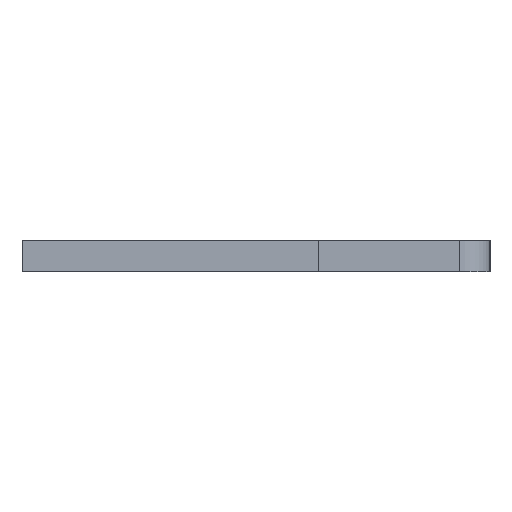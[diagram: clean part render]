
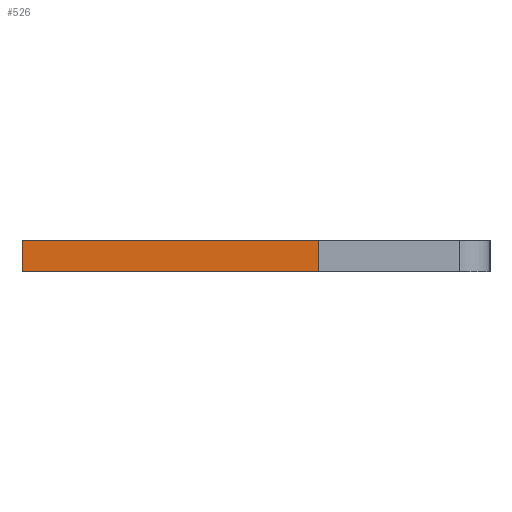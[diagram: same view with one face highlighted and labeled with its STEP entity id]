
A CAD part, left-side view. The second image highlights one B-rep face of the part: STEP entity #526.
In plain terms, the highlighted face is planar.
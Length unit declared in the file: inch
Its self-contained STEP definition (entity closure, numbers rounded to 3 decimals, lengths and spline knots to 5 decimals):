
#47 = ORIENTED_EDGE ( 'NONE', *, *, #707, .T. ) ;
#211 = CARTESIAN_POINT ( 'NONE',  ( 0.01, 0.15, -0.04 ) ) ;
#307 = LINE ( 'NONE', #580, #991 ) ;
#355 = DIRECTION ( 'NONE',  ( -1., 0., 0. ) ) ;
#461 = EDGE_CURVE ( 'NONE', #1667, #1750, #1270, .T. ) ;
#514 = LINE ( 'NONE', #666, #1450 ) ;
#526 = ADVANCED_FACE ( 'NONE', ( #1645 ), #1375, .F. ) ;
#580 = CARTESIAN_POINT ( 'NONE',  ( 0.01, -0.04, -0.04 ) ) ;
#611 = LINE ( 'NONE', #1779, #1661 ) ;
#666 = CARTESIAN_POINT ( 'NONE',  ( -0.01, 0.15, -0.04 ) ) ;
#679 = EDGE_LOOP ( 'NONE', ( #47, #1548, #1771, #1090 ) ) ;
#707 = EDGE_CURVE ( 'NONE', #1342, #1750, #514, .T. ) ;
#747 = DIRECTION ( 'NONE',  ( 0., 1., 0. ) ) ;
#776 = DIRECTION ( 'NONE',  ( 1., 0., 0. ) ) ;
#801 = DIRECTION ( 'NONE',  ( 0., 0., 1. ) ) ;
#887 = DIRECTION ( 'NONE',  ( -1., 0., 0. ) ) ;
#944 = VERTEX_POINT ( 'NONE', #1073 ) ;
#991 = VECTOR ( 'NONE', #887, 39.37008 ) ;
#1073 = CARTESIAN_POINT ( 'NONE',  ( 0.01, -0.04, -0.04 ) ) ;
#1090 = ORIENTED_EDGE ( 'NONE', *, *, #1600, .T. ) ;
#1099 = CARTESIAN_POINT ( 'NONE',  ( -0.01, -0.04, -0.04 ) ) ;
#1116 = EDGE_CURVE ( 'NONE', #944, #1667, #611, .T. ) ;
#1264 = DIRECTION ( 'NONE',  ( 0., 1., 0. ) ) ;
#1270 = LINE ( 'NONE', #211, #1506 ) ;
#1309 = AXIS2_PLACEMENT_3D ( 'NONE', #1521, #801, #776 ) ;
#1342 = VERTEX_POINT ( 'NONE', #1099 ) ;
#1375 = PLANE ( 'NONE',  #1309 ) ;
#1450 = VECTOR ( 'NONE', #1264, 39.37008 ) ;
#1470 = CARTESIAN_POINT ( 'NONE',  ( 0.01, 0.15, -0.04 ) ) ;
#1506 = VECTOR ( 'NONE', #355, 39.37008 ) ;
#1521 = CARTESIAN_POINT ( 'NONE',  ( 0.01, 0.15, -0.04 ) ) ;
#1548 = ORIENTED_EDGE ( 'NONE', *, *, #461, .F. ) ;
#1600 = EDGE_CURVE ( 'NONE', #944, #1342, #307, .T. ) ;
#1645 = FACE_OUTER_BOUND ( 'NONE', #679, .T. ) ;
#1661 = VECTOR ( 'NONE', #747, 39.37008 ) ;
#1667 = VERTEX_POINT ( 'NONE', #1470 ) ;
#1750 = VERTEX_POINT ( 'NONE', #1770 ) ;
#1770 = CARTESIAN_POINT ( 'NONE',  ( -0.01, 0.15, -0.04 ) ) ;
#1771 = ORIENTED_EDGE ( 'NONE', *, *, #1116, .F. ) ;
#1779 = CARTESIAN_POINT ( 'NONE',  ( 0.01, 0.15, -0.04 ) ) ;
